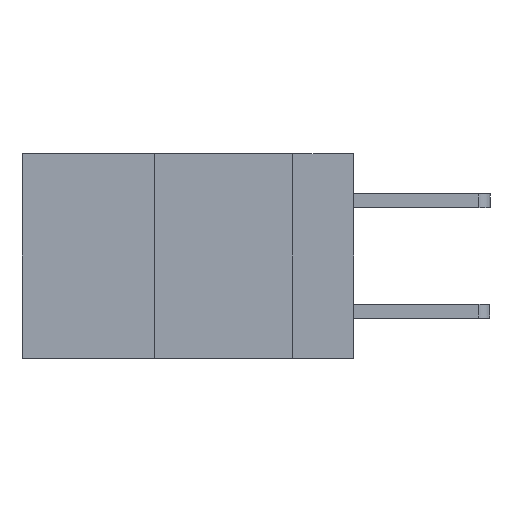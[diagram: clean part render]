
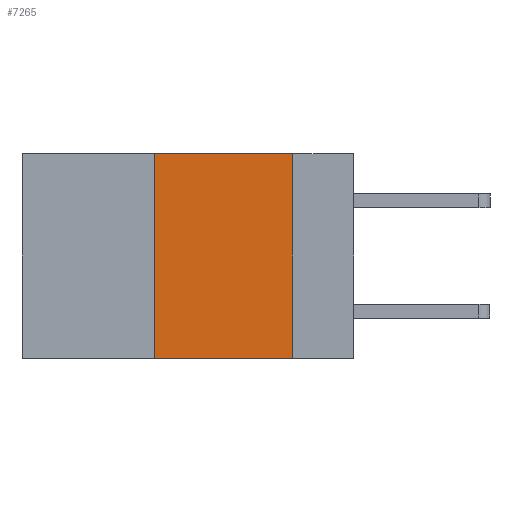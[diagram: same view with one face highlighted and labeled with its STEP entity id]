
A CAD part, left-side view. The second image highlights one B-rep face of the part: STEP entity #7265.
In plain terms, the highlighted planar face has unit normal (-1, 0, 0).
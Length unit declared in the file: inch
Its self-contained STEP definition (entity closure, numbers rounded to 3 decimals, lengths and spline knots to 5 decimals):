
#152 = AXIS2_PLACEMENT_3D ( 'NONE', #12050, #1794, #886 ) ;
#371 = CARTESIAN_POINT ( 'NONE',  ( 0., 0.36, -0.37 ) ) ;
#582 = LINE ( 'NONE', #5944, #3828 ) ;
#635 = ORIENTED_EDGE ( 'NONE', *, *, #4394, .F. ) ;
#677 = LINE ( 'NONE', #1640, #10529 ) ;
#886 = DIRECTION ( 'NONE',  ( 0., 0., -1. ) ) ;
#1640 = CARTESIAN_POINT ( 'NONE',  ( 0., 0.11, 0. ) ) ;
#1794 = DIRECTION ( 'NONE',  ( 1., 0., 0. ) ) ;
#1903 = VECTOR ( 'NONE', #1912, 39.37008 ) ;
#1912 = DIRECTION ( 'NONE',  ( 0., -1., 0. ) ) ;
#1956 = CARTESIAN_POINT ( 'NONE',  ( 0., 0.36, 0. ) ) ;
#2324 = LINE ( 'NONE', #11261, #1903 ) ;
#2344 = EDGE_CURVE ( 'NONE', #4099, #8876, #9433, .T. ) ;
#2383 = ORIENTED_EDGE ( 'NONE', *, *, #5504, .T. ) ;
#3072 = ORIENTED_EDGE ( 'NONE', *, *, #2344, .F. ) ;
#3480 = DIRECTION ( 'NONE',  ( 0., 0., -1. ) ) ;
#3828 = VECTOR ( 'NONE', #4295, 39.37008 ) ;
#3829 = VERTEX_POINT ( 'NONE', #10283 ) ;
#4099 = VERTEX_POINT ( 'NONE', #1956 ) ;
#4295 = DIRECTION ( 'NONE',  ( 0., 0., 1. ) ) ;
#4371 = PLANE ( 'NONE',  #152 ) ;
#4394 = EDGE_CURVE ( 'NONE', #9253, #4099, #582, .T. ) ;
#4552 = FACE_OUTER_BOUND ( 'NONE', #8648, .T. ) ;
#4749 = DIRECTION ( 'NONE',  ( 0., -1., 0. ) ) ;
#5116 = EDGE_CURVE ( 'NONE', #8876, #3829, #677, .T. ) ;
#5504 = EDGE_CURVE ( 'NONE', #9253, #3829, #2324, .T. ) ;
#5864 = CARTESIAN_POINT ( 'NONE',  ( 0., 0.6, 0. ) ) ;
#5944 = CARTESIAN_POINT ( 'NONE',  ( 0., 0.36, 0. ) ) ;
#6171 = ORIENTED_EDGE ( 'NONE', *, *, #5116, .F. ) ;
#7265 = ADVANCED_FACE ( 'NONE', ( #4552 ), #4371, .F. ) ;
#8648 = EDGE_LOOP ( 'NONE', ( #6171, #3072, #635, #2383 ) ) ;
#8876 = VERTEX_POINT ( 'NONE', #10629 ) ;
#9253 = VERTEX_POINT ( 'NONE', #371 ) ;
#9433 = LINE ( 'NONE', #5864, #9513 ) ;
#9513 = VECTOR ( 'NONE', #4749, 39.37008 ) ;
#10283 = CARTESIAN_POINT ( 'NONE',  ( 0., 0.11, -0.37 ) ) ;
#10529 = VECTOR ( 'NONE', #3480, 39.37008 ) ;
#10629 = CARTESIAN_POINT ( 'NONE',  ( 0., 0.11, 0. ) ) ;
#11261 = CARTESIAN_POINT ( 'NONE',  ( 0., 0.6, -0.37 ) ) ;
#12050 = CARTESIAN_POINT ( 'NONE',  ( 0., 0.6, 0. ) ) ;
